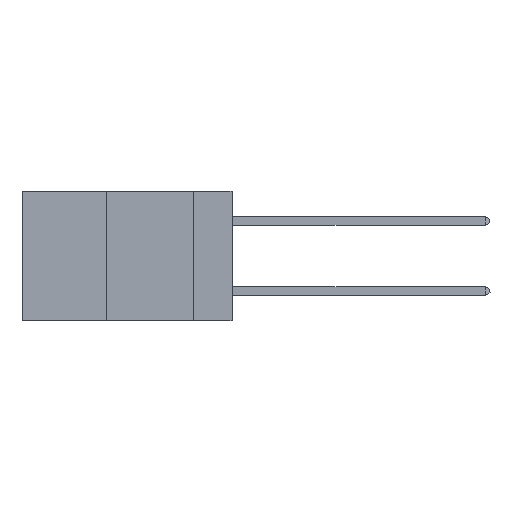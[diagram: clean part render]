
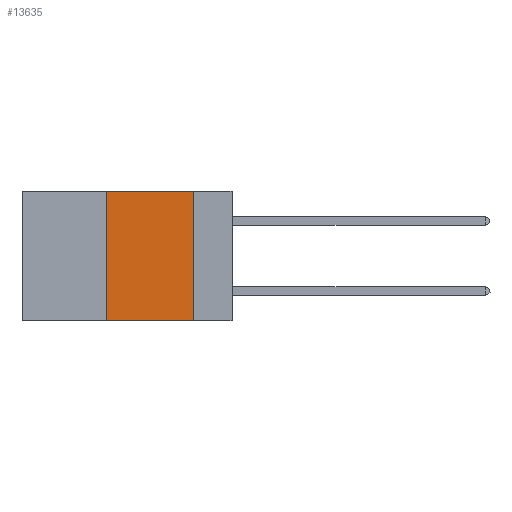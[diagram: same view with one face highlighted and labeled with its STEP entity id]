
A CAD part, left-side view. The second image highlights one B-rep face of the part: STEP entity #13635.
In plain terms, the highlighted planar face has unit normal (-1, 0, 0).
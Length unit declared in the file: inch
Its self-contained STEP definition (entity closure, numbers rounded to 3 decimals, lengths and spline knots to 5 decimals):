
#169 = LINE ( 'NONE', #1140, #11675 ) ;
#419 = ORIENTED_EDGE ( 'NONE', *, *, #4126, .F. ) ;
#718 = AXIS2_PLACEMENT_3D ( 'NONE', #4627, #6583, #5673 ) ;
#964 = EDGE_CURVE ( 'NONE', #1327, #6060, #1660, .T. ) ;
#1105 = VECTOR ( 'NONE', #10212, 39.37008 ) ;
#1140 = CARTESIAN_POINT ( 'NONE',  ( 0., 0.6, 0. ) ) ;
#1203 = CARTESIAN_POINT ( 'NONE',  ( 0., 0.36, -0.37 ) ) ;
#1327 = VERTEX_POINT ( 'NONE', #1203 ) ;
#1660 = LINE ( 'NONE', #5922, #1105 ) ;
#2253 = CARTESIAN_POINT ( 'NONE',  ( 0., 0.11, 0. ) ) ;
#2404 = CARTESIAN_POINT ( 'NONE',  ( 0., 0.36, 0. ) ) ;
#2718 = CARTESIAN_POINT ( 'NONE',  ( 0., 0.11, -0.37 ) ) ;
#2778 = VERTEX_POINT ( 'NONE', #2718 ) ;
#3563 = FACE_OUTER_BOUND ( 'NONE', #9874, .T. ) ;
#4126 = EDGE_CURVE ( 'NONE', #7773, #2778, #7927, .T. ) ;
#4353 = DIRECTION ( 'NONE',  ( 0., -1., 0. ) ) ;
#4627 = CARTESIAN_POINT ( 'NONE',  ( 0., 0.6, 0. ) ) ;
#5502 = LINE ( 'NONE', #13081, #8269 ) ;
#5630 = EDGE_CURVE ( 'NONE', #1327, #2778, #5502, .T. ) ;
#5673 = DIRECTION ( 'NONE',  ( 0., 0., -1. ) ) ;
#5922 = CARTESIAN_POINT ( 'NONE',  ( 0., 0.36, 0. ) ) ;
#6060 = VERTEX_POINT ( 'NONE', #2404 ) ;
#6583 = DIRECTION ( 'NONE',  ( 1., 0., 0. ) ) ;
#6661 = DIRECTION ( 'NONE',  ( 0., 0., -1. ) ) ;
#7207 = ORIENTED_EDGE ( 'NONE', *, *, #5630, .T. ) ;
#7773 = VERTEX_POINT ( 'NONE', #2253 ) ;
#7927 = LINE ( 'NONE', #12141, #12862 ) ;
#8269 = VECTOR ( 'NONE', #9798, 39.37008 ) ;
#9798 = DIRECTION ( 'NONE',  ( 0., -1., 0. ) ) ;
#9874 = EDGE_LOOP ( 'NONE', ( #419, #12525, #12782, #7207 ) ) ;
#9894 = PLANE ( 'NONE',  #718 ) ;
#10212 = DIRECTION ( 'NONE',  ( 0., 0., 1. ) ) ;
#11675 = VECTOR ( 'NONE', #4353, 39.37008 ) ;
#12141 = CARTESIAN_POINT ( 'NONE',  ( 0., 0.11, 0. ) ) ;
#12525 = ORIENTED_EDGE ( 'NONE', *, *, #13412, .F. ) ;
#12782 = ORIENTED_EDGE ( 'NONE', *, *, #964, .F. ) ;
#12862 = VECTOR ( 'NONE', #6661, 39.37008 ) ;
#13081 = CARTESIAN_POINT ( 'NONE',  ( 0., 0.6, -0.37 ) ) ;
#13412 = EDGE_CURVE ( 'NONE', #6060, #7773, #169, .T. ) ;
#13635 = ADVANCED_FACE ( 'NONE', ( #3563 ), #9894, .F. ) ;
